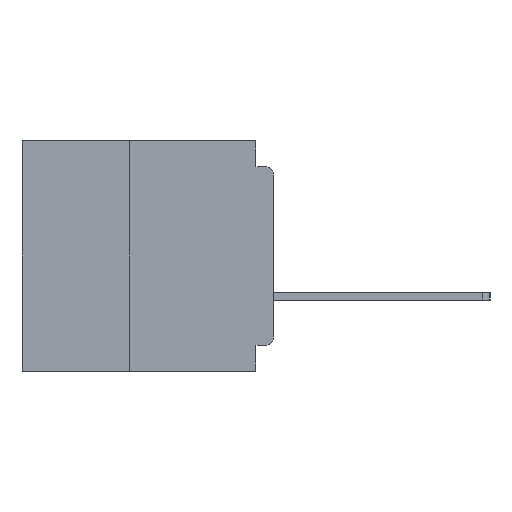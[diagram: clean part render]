
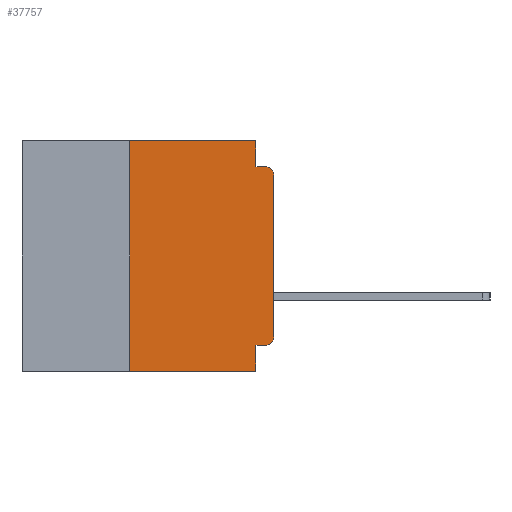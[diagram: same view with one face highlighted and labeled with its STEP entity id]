
A CAD part, left-side view. The second image highlights one B-rep face of the part: STEP entity #37757.
In plain terms, the highlighted planar face has unit normal (-1, 0, 0).
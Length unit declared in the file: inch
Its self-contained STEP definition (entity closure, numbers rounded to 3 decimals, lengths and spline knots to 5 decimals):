
#290 = DIRECTION ( 'NONE',  ( -1., 0., 0. ) ) ;
#2207 = CARTESIAN_POINT ( 'NONE',  ( 0., 0.015, -0.06 ) ) ;
#3100 = EDGE_CURVE ( 'NONE', #35870, #18727, #31706, .T. ) ;
#4129 = CARTESIAN_POINT ( 'NONE',  ( 0., 0.015, -0.355 ) ) ;
#5347 = ORIENTED_EDGE ( 'NONE', *, *, #42056, .T. ) ;
#5419 = LINE ( 'NONE', #10348, #25536 ) ;
#5461 = CARTESIAN_POINT ( 'NONE',  ( 0., 0.031, -0.045 ) ) ;
#5941 = DIRECTION ( 'NONE',  ( 0., 0., -1. ) ) ;
#6281 = VERTEX_POINT ( 'NONE', #41528 ) ;
#6973 = ORIENTED_EDGE ( 'NONE', *, *, #36878, .F. ) ;
#7217 = EDGE_CURVE ( 'NONE', #18727, #35689, #45338, .T. ) ;
#7553 = EDGE_CURVE ( 'NONE', #14705, #41877, #40039, .T. ) ;
#7922 = VERTEX_POINT ( 'NONE', #36371 ) ;
#8126 = DIRECTION ( 'NONE',  ( 1., 0., 0. ) ) ;
#8478 = VERTEX_POINT ( 'NONE', #5461 ) ;
#8942 = CIRCLE ( 'NONE', #31112, 0.015 ) ;
#9023 = ORIENTED_EDGE ( 'NONE', *, *, #7217, .F. ) ;
#9231 = CARTESIAN_POINT ( 'NONE',  ( 0., 0.031, 0. ) ) ;
#9565 = AXIS2_PLACEMENT_3D ( 'NONE', #2207, #28598, #5941 ) ;
#10348 = CARTESIAN_POINT ( 'NONE',  ( 0., 0., 0. ) ) ;
#11797 = LINE ( 'NONE', #31486, #28385 ) ;
#12188 = CIRCLE ( 'NONE', #9565, 0.015 ) ;
#12505 = ORIENTED_EDGE ( 'NONE', *, *, #39412, .T. ) ;
#13030 = CARTESIAN_POINT ( 'NONE',  ( 0., 0.031, -0.355 ) ) ;
#13572 = EDGE_CURVE ( 'NONE', #14705, #6281, #8942, .T. ) ;
#14390 = FACE_OUTER_BOUND ( 'NONE', #26379, .T. ) ;
#14705 = VERTEX_POINT ( 'NONE', #4129 ) ;
#15652 = EDGE_CURVE ( 'NONE', #35689, #8478, #44158, .T. ) ;
#16612 = CARTESIAN_POINT ( 'NONE',  ( 0., 0., -0.355 ) ) ;
#17822 = VERTEX_POINT ( 'NONE', #33463 ) ;
#18256 = LINE ( 'NONE', #23495, #37167 ) ;
#18727 = VERTEX_POINT ( 'NONE', #47747 ) ;
#20120 = ORIENTED_EDGE ( 'NONE', *, *, #40489, .F. ) ;
#20447 = CARTESIAN_POINT ( 'NONE',  ( 0., 0., -0.06 ) ) ;
#20808 = DIRECTION ( 'NONE',  ( 0., -1., 0. ) ) ;
#21354 = CARTESIAN_POINT ( 'NONE',  ( 0., 0.031, -0.4 ) ) ;
#21501 = DIRECTION ( 'NONE',  ( 0., 0., -1. ) ) ;
#21800 = DIRECTION ( 'NONE',  ( 0., 0., 1. ) ) ;
#22133 = VERTEX_POINT ( 'NONE', #20447 ) ;
#22866 = CARTESIAN_POINT ( 'NONE',  ( 0., 0.015, -0.34 ) ) ;
#23495 = CARTESIAN_POINT ( 'NONE',  ( 0., 0., -0.045 ) ) ;
#25536 = VECTOR ( 'NONE', #21800, 39.37008 ) ;
#26379 = EDGE_LOOP ( 'NONE', ( #5347, #48391, #20120, #31892, #9023, #42618, #12505, #6973, #26447, #32895 ) ) ;
#26447 = ORIENTED_EDGE ( 'NONE', *, *, #7553, .F. ) ;
#26693 = DIRECTION ( 'NONE',  ( 0., 0., -1. ) ) ;
#26728 = CARTESIAN_POINT ( 'NONE',  ( 0., 0.25, -0.4 ) ) ;
#26972 = LINE ( 'NONE', #21354, #45768 ) ;
#27307 = DIRECTION ( 'NONE',  ( 0., -1., 0. ) ) ;
#28385 = VECTOR ( 'NONE', #35261, 39.37008 ) ;
#28598 = DIRECTION ( 'NONE',  ( -1., 0., 0. ) ) ;
#29988 = VECTOR ( 'NONE', #37732, 39.37008 ) ;
#30520 = VECTOR ( 'NONE', #44818, 39.37008 ) ;
#30797 = CARTESIAN_POINT ( 'NONE',  ( 0., 0.437, 0. ) ) ;
#31112 = AXIS2_PLACEMENT_3D ( 'NONE', #22866, #290, #26693 ) ;
#31316 = EDGE_CURVE ( 'NONE', #22133, #17822, #12188, .T. ) ;
#31486 = CARTESIAN_POINT ( 'NONE',  ( 0., 0.437, -0.4 ) ) ;
#31706 = LINE ( 'NONE', #41037, #30520 ) ;
#31892 = ORIENTED_EDGE ( 'NONE', *, *, #15652, .F. ) ;
#32895 = ORIENTED_EDGE ( 'NONE', *, *, #13572, .T. ) ;
#33463 = CARTESIAN_POINT ( 'NONE',  ( 0., 0.015, -0.045 ) ) ;
#34090 = VECTOR ( 'NONE', #43259, 39.37008 ) ;
#34550 = DIRECTION ( 'NONE',  ( 0., 0., -1. ) ) ;
#35261 = DIRECTION ( 'NONE',  ( 0., -1., 0. ) ) ;
#35323 = VECTOR ( 'NONE', #20808, 39.37008 ) ;
#35689 = VERTEX_POINT ( 'NONE', #48253 ) ;
#35870 = VERTEX_POINT ( 'NONE', #26728 ) ;
#36371 = CARTESIAN_POINT ( 'NONE',  ( 0., 0.031, -0.4 ) ) ;
#36878 = EDGE_CURVE ( 'NONE', #41877, #7922, #26972, .T. ) ;
#37167 = VECTOR ( 'NONE', #27307, 39.37008 ) ;
#37732 = DIRECTION ( 'NONE',  ( 0., 1., 0. ) ) ;
#37757 = ADVANCED_FACE ( 'NONE', ( #14390 ), #45762, .F. ) ;
#39412 = EDGE_CURVE ( 'NONE', #35870, #7922, #11797, .T. ) ;
#40039 = LINE ( 'NONE', #16612, #29988 ) ;
#40489 = EDGE_CURVE ( 'NONE', #8478, #17822, #18256, .T. ) ;
#41037 = CARTESIAN_POINT ( 'NONE',  ( 0., 0.25, -0.4 ) ) ;
#41528 = CARTESIAN_POINT ( 'NONE',  ( 0., 0., -0.34 ) ) ;
#41877 = VERTEX_POINT ( 'NONE', #13030 ) ;
#42056 = EDGE_CURVE ( 'NONE', #6281, #22133, #5419, .T. ) ;
#42618 = ORIENTED_EDGE ( 'NONE', *, *, #3100, .F. ) ;
#42697 = AXIS2_PLACEMENT_3D ( 'NONE', #30797, #8126, #34550 ) ;
#43259 = DIRECTION ( 'NONE',  ( 0., 0., -1. ) ) ;
#44158 = LINE ( 'NONE', #9231, #34090 ) ;
#44818 = DIRECTION ( 'NONE',  ( 0., 0., 1. ) ) ;
#45338 = LINE ( 'NONE', #47143, #35323 ) ;
#45762 = PLANE ( 'NONE',  #42697 ) ;
#45768 = VECTOR ( 'NONE', #21501, 39.37008 ) ;
#47143 = CARTESIAN_POINT ( 'NONE',  ( 0., 0.437, 0. ) ) ;
#47747 = CARTESIAN_POINT ( 'NONE',  ( 0., 0.25, 0. ) ) ;
#48253 = CARTESIAN_POINT ( 'NONE',  ( 0., 0.031, 0. ) ) ;
#48391 = ORIENTED_EDGE ( 'NONE', *, *, #31316, .T. ) ;
